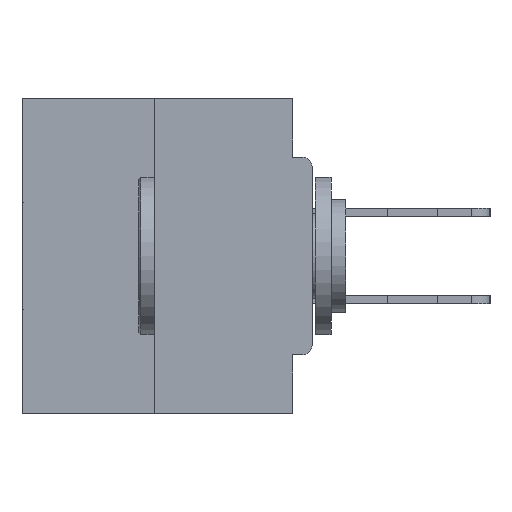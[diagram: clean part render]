
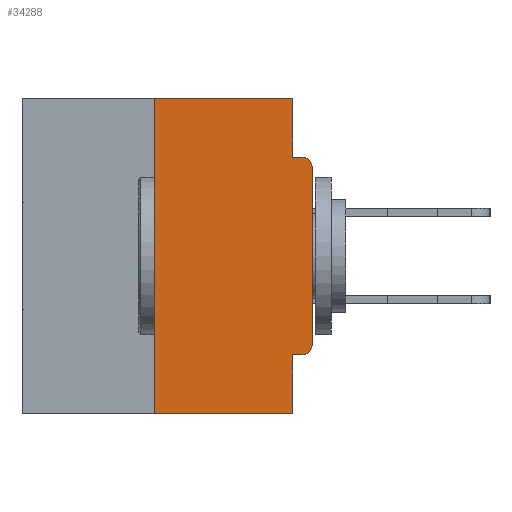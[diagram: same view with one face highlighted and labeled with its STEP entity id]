
A CAD part, left-side view. The second image highlights one B-rep face of the part: STEP entity #34288.
In plain terms, the highlighted planar face has unit normal (-1, 0, 0).
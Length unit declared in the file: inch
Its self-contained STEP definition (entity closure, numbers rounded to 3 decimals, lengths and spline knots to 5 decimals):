
#757 = CARTESIAN_POINT ( 'NONE',  ( 0., 0.015, -0.0935 ) ) ;
#1750 = VECTOR ( 'NONE', #33620, 39.37008 ) ;
#2185 = CIRCLE ( 'NONE', #35906, 0.015 ) ;
#2551 = DIRECTION ( 'NONE',  ( 0., -1., 0. ) ) ;
#3340 = CARTESIAN_POINT ( 'NONE',  ( 0., 0.015, -0.4065 ) ) ;
#3542 = VERTEX_POINT ( 'NONE', #27800 ) ;
#3558 = EDGE_CURVE ( 'NONE', #9320, #20434, #6804, .T. ) ;
#4513 = CARTESIAN_POINT ( 'NONE',  ( 0., 0.031, 0. ) ) ;
#4669 = VERTEX_POINT ( 'NONE', #34249 ) ;
#4911 = VECTOR ( 'NONE', #6958, 39.37008 ) ;
#5188 = VECTOR ( 'NONE', #15860, 39.37008 ) ;
#5418 = LINE ( 'NONE', #4513, #4911 ) ;
#5791 = CARTESIAN_POINT ( 'NONE',  ( 0., 0.25, 0. ) ) ;
#6804 = LINE ( 'NONE', #34257, #31022 ) ;
#6958 = DIRECTION ( 'NONE',  ( 0., 0., -1. ) ) ;
#7075 = AXIS2_PLACEMENT_3D ( 'NONE', #8029, #20605, #14624 ) ;
#7668 = EDGE_CURVE ( 'NONE', #20434, #10814, #33809, .T. ) ;
#8029 = CARTESIAN_POINT ( 'NONE',  ( 0., 0.46, 0. ) ) ;
#8723 = CARTESIAN_POINT ( 'NONE',  ( 0., 0.25, 0. ) ) ;
#8733 = CARTESIAN_POINT ( 'NONE',  ( 0., 0.015, -0.3915 ) ) ;
#8961 = EDGE_LOOP ( 'NONE', ( #32325, #30803, #11234, #17110, #11103, #10080, #34793, #15607, #27663, #9479 ) ) ;
#9320 = VERTEX_POINT ( 'NONE', #3340 ) ;
#9326 = CARTESIAN_POINT ( 'NONE',  ( 0., 0.031, -0.5 ) ) ;
#9453 = VECTOR ( 'NONE', #24624, 39.37008 ) ;
#9479 = ORIENTED_EDGE ( 'NONE', *, *, #11717, .F. ) ;
#9850 = VERTEX_POINT ( 'NONE', #26806 ) ;
#10080 = ORIENTED_EDGE ( 'NONE', *, *, #26165, .T. ) ;
#10669 = CARTESIAN_POINT ( 'NONE',  ( 0., 0.031, -0.4065 ) ) ;
#10814 = VERTEX_POINT ( 'NONE', #34883 ) ;
#11103 = ORIENTED_EDGE ( 'NONE', *, *, #3558, .F. ) ;
#11179 = CIRCLE ( 'NONE', #37518, 0.015 ) ;
#11234 = ORIENTED_EDGE ( 'NONE', *, *, #26127, .T. ) ;
#11717 = EDGE_CURVE ( 'NONE', #27062, #4669, #5418, .T. ) ;
#12039 = FACE_OUTER_BOUND ( 'NONE', #8961, .T. ) ;
#13024 = LINE ( 'NONE', #23885, #39189 ) ;
#13509 = DIRECTION ( 'NONE',  ( 0., 0., -1. ) ) ;
#14027 = LINE ( 'NONE', #18026, #1750 ) ;
#14624 = DIRECTION ( 'NONE',  ( 0., 0., -1. ) ) ;
#15040 = DIRECTION ( 'NONE',  ( -1., 0., 0. ) ) ;
#15607 = ORIENTED_EDGE ( 'NONE', *, *, #37951, .T. ) ;
#15860 = DIRECTION ( 'NONE',  ( 0., -1., 0. ) ) ;
#16419 = VERTEX_POINT ( 'NONE', #5791 ) ;
#17110 = ORIENTED_EDGE ( 'NONE', *, *, #7668, .F. ) ;
#18026 = CARTESIAN_POINT ( 'NONE',  ( 0., 0., -0.0935 ) ) ;
#18626 = CARTESIAN_POINT ( 'NONE',  ( 0., 0., -0.3915 ) ) ;
#19052 = CARTESIAN_POINT ( 'NONE',  ( 0., 0.46, 0. ) ) ;
#19962 = VECTOR ( 'NONE', #2551, 39.37008 ) ;
#20434 = VERTEX_POINT ( 'NONE', #10669 ) ;
#20605 = DIRECTION ( 'NONE',  ( 1., 0., 0. ) ) ;
#21142 = VERTEX_POINT ( 'NONE', #18626 ) ;
#21151 = CARTESIAN_POINT ( 'NONE',  ( 0., 0.46, -0.5 ) ) ;
#22194 = DIRECTION ( 'NONE',  ( 0., 0., -1. ) ) ;
#23885 = CARTESIAN_POINT ( 'NONE',  ( 0., 0., 0. ) ) ;
#24624 = DIRECTION ( 'NONE',  ( 0., 0., 1. ) ) ;
#25534 = EDGE_CURVE ( 'NONE', #4669, #30450, #14027, .T. ) ;
#26127 = EDGE_CURVE ( 'NONE', #9850, #10814, #34794, .T. ) ;
#26165 = EDGE_CURVE ( 'NONE', #9320, #21142, #2185, .T. ) ;
#26536 = DIRECTION ( 'NONE',  ( -1., 0., 0. ) ) ;
#26806 = CARTESIAN_POINT ( 'NONE',  ( 0., 0.25, -0.5 ) ) ;
#27062 = VERTEX_POINT ( 'NONE', #37970 ) ;
#27663 = ORIENTED_EDGE ( 'NONE', *, *, #25534, .F. ) ;
#27800 = CARTESIAN_POINT ( 'NONE',  ( 0., 0., -0.1085 ) ) ;
#28661 = EDGE_CURVE ( 'NONE', #21142, #3542, #13024, .T. ) ;
#30076 = DIRECTION ( 'NONE',  ( 0., 0., 1. ) ) ;
#30222 = EDGE_CURVE ( 'NONE', #9850, #16419, #33164, .T. ) ;
#30450 = VERTEX_POINT ( 'NONE', #757 ) ;
#30803 = ORIENTED_EDGE ( 'NONE', *, *, #30222, .F. ) ;
#31022 = VECTOR ( 'NONE', #34123, 39.37008 ) ;
#31405 = VECTOR ( 'NONE', #22194, 39.37008 ) ;
#32325 = ORIENTED_EDGE ( 'NONE', *, *, #33517, .F. ) ;
#33164 = LINE ( 'NONE', #8723, #9453 ) ;
#33380 = LINE ( 'NONE', #19052, #5188 ) ;
#33517 = EDGE_CURVE ( 'NONE', #16419, #27062, #33380, .T. ) ;
#33620 = DIRECTION ( 'NONE',  ( 0., -1., 0. ) ) ;
#33683 = PLANE ( 'NONE',  #7075 ) ;
#33809 = LINE ( 'NONE', #9326, #31405 ) ;
#34123 = DIRECTION ( 'NONE',  ( 0., 1., 0. ) ) ;
#34249 = CARTESIAN_POINT ( 'NONE',  ( 0., 0.031, -0.0935 ) ) ;
#34257 = CARTESIAN_POINT ( 'NONE',  ( 0., 0., -0.4065 ) ) ;
#34288 = ADVANCED_FACE ( 'NONE', ( #12039 ), #33683, .F. ) ;
#34793 = ORIENTED_EDGE ( 'NONE', *, *, #28661, .T. ) ;
#34794 = LINE ( 'NONE', #21151, #19962 ) ;
#34883 = CARTESIAN_POINT ( 'NONE',  ( 0., 0.031, -0.5 ) ) ;
#35761 = CARTESIAN_POINT ( 'NONE',  ( 0., 0.015, -0.1085 ) ) ;
#35906 = AXIS2_PLACEMENT_3D ( 'NONE', #8733, #15040, #40010 ) ;
#37518 = AXIS2_PLACEMENT_3D ( 'NONE', #35761, #26536, #13509 ) ;
#37951 = EDGE_CURVE ( 'NONE', #3542, #30450, #11179, .T. ) ;
#37970 = CARTESIAN_POINT ( 'NONE',  ( 0., 0.031, 0. ) ) ;
#39189 = VECTOR ( 'NONE', #30076, 39.37008 ) ;
#40010 = DIRECTION ( 'NONE',  ( 0., 0., -1. ) ) ;
